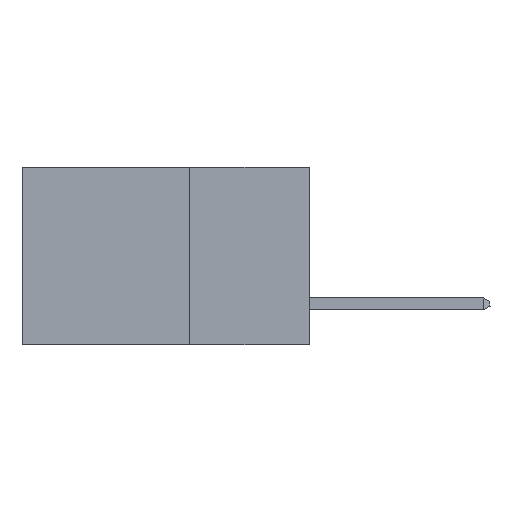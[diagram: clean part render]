
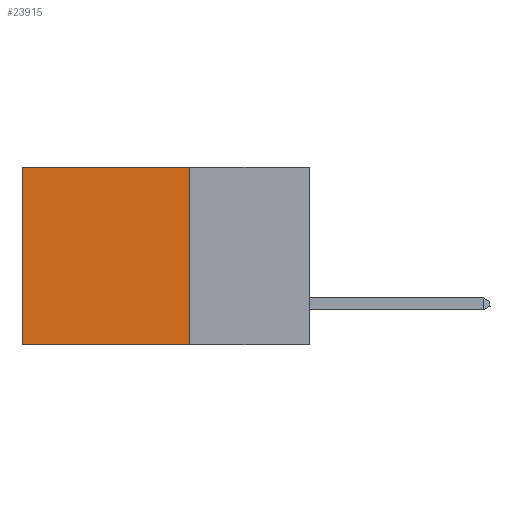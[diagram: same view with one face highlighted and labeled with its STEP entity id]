
A CAD part, left-side view. The second image highlights one B-rep face of the part: STEP entity #23915.
In plain terms, the highlighted planar face has unit normal (-1, 0, 0).
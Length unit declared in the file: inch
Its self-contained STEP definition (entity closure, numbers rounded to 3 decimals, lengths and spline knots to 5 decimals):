
#1949 = CARTESIAN_POINT ( 'NONE',  ( 0.2875, 0.25, 0. ) ) ;
#2319 = EDGE_CURVE ( 'NONE', #30108, #21927, #39002, .T. ) ;
#3075 = VECTOR ( 'NONE', #18703, 39.37008 ) ;
#3268 = VERTEX_POINT ( 'NONE', #1949 ) ;
#6793 = PLANE ( 'NONE',  #24218 ) ;
#8487 = CARTESIAN_POINT ( 'NONE',  ( 0.2875, 0.6, 0. ) ) ;
#8851 = EDGE_LOOP ( 'NONE', ( #29930, #16969, #11394, #16128 ) ) ;
#8968 = LINE ( 'NONE', #28744, #17649 ) ;
#8976 = DIRECTION ( 'NONE',  ( 0., 0., -1. ) ) ;
#9269 = EDGE_CURVE ( 'NONE', #21443, #21927, #19883, .T. ) ;
#11394 = ORIENTED_EDGE ( 'NONE', *, *, #29246, .F. ) ;
#13000 = DIRECTION ( 'NONE',  ( 0., 0., -1. ) ) ;
#14889 = LINE ( 'NONE', #38326, #3075 ) ;
#16128 = ORIENTED_EDGE ( 'NONE', *, *, #25513, .T. ) ;
#16540 = FACE_OUTER_BOUND ( 'NONE', #8851, .T. ) ;
#16969 = ORIENTED_EDGE ( 'NONE', *, *, #2319, .F. ) ;
#17518 = DIRECTION ( 'NONE',  ( 0., 0., -1. ) ) ;
#17649 = VECTOR ( 'NONE', #8976, 39.37008 ) ;
#17770 = VECTOR ( 'NONE', #17518, 39.37008 ) ;
#18353 = CARTESIAN_POINT ( 'NONE',  ( 0.2875, 0.25, -0.37 ) ) ;
#18703 = DIRECTION ( 'NONE',  ( 0., 1., 0. ) ) ;
#18806 = DIRECTION ( 'NONE',  ( 0., 1., 0. ) ) ;
#18950 = CARTESIAN_POINT ( 'NONE',  ( 0.2875, 0.25, -0.37 ) ) ;
#19883 = LINE ( 'NONE', #35810, #17770 ) ;
#21443 = VERTEX_POINT ( 'NONE', #8487 ) ;
#21927 = VERTEX_POINT ( 'NONE', #23954 ) ;
#23085 = DIRECTION ( 'NONE',  ( 1., 0., 0. ) ) ;
#23915 = ADVANCED_FACE ( 'NONE', ( #16540 ), #6793, .F. ) ;
#23954 = CARTESIAN_POINT ( 'NONE',  ( 0.2875, 0.6, -0.37 ) ) ;
#24218 = AXIS2_PLACEMENT_3D ( 'NONE', #39537, #23085, #13000 ) ;
#25513 = EDGE_CURVE ( 'NONE', #3268, #21443, #14889, .T. ) ;
#28744 = CARTESIAN_POINT ( 'NONE',  ( 0.2875, 0.25, 0. ) ) ;
#29246 = EDGE_CURVE ( 'NONE', #3268, #30108, #8968, .T. ) ;
#29930 = ORIENTED_EDGE ( 'NONE', *, *, #9269, .T. ) ;
#30108 = VERTEX_POINT ( 'NONE', #18353 ) ;
#33337 = VECTOR ( 'NONE', #18806, 39.37008 ) ;
#35810 = CARTESIAN_POINT ( 'NONE',  ( 0.2875, 0.6, 0. ) ) ;
#38326 = CARTESIAN_POINT ( 'NONE',  ( 0.2875, 0.25, 0. ) ) ;
#39002 = LINE ( 'NONE', #18950, #33337 ) ;
#39537 = CARTESIAN_POINT ( 'NONE',  ( 0.2875, 0.25, 0. ) ) ;
